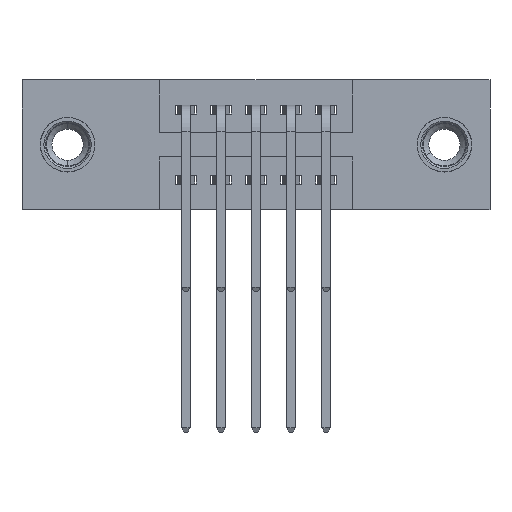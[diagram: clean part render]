
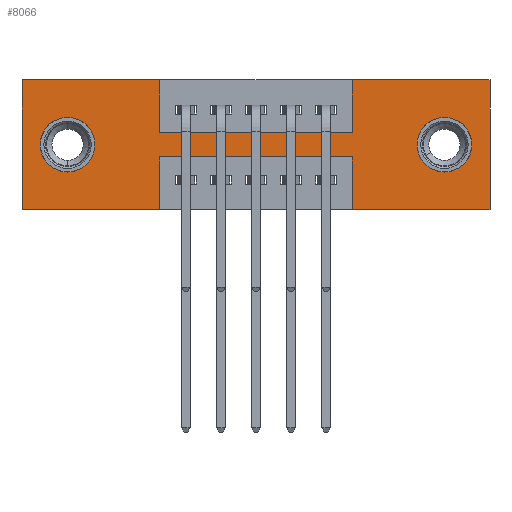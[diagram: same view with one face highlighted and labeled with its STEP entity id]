
A CAD part, front view. The second image highlights one B-rep face of the part: STEP entity #8066.
In plain terms, the highlighted planar face has unit normal (0, -1, 0).
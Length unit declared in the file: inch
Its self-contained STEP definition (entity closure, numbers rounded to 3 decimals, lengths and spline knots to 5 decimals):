
#124 = CARTESIAN_POINT ( 'NONE',  ( 0.13, 0., -0.107 ) ) ;
#285 = EDGE_CURVE ( 'NONE', #5624, #4382, #314, .T. ) ;
#314 = LINE ( 'NONE', #6345, #8420 ) ;
#387 = ORIENTED_EDGE ( 'NONE', *, *, #9266, .F. ) ;
#446 = CARTESIAN_POINT ( 'NONE',  ( 1.335, 0., 0. ) ) ;
#456 = VECTOR ( 'NONE', #890, 39.37008 ) ;
#556 = EDGE_CURVE ( 'NONE', #1943, #1924, #5445, .T. ) ;
#660 = CARTESIAN_POINT ( 'NONE',  ( 0.13, 0., -0.185 ) ) ;
#846 = LINE ( 'NONE', #3126, #1568 ) ;
#890 = DIRECTION ( 'NONE',  ( 0., 0., -1. ) ) ;
#943 = CIRCLE ( 'NONE', #5551, 0.078 ) ;
#991 = AXIS2_PLACEMENT_3D ( 'NONE', #660, #4293, #2564 ) ;
#1037 = CARTESIAN_POINT ( 'NONE',  ( 1.205, 0., -0.107 ) ) ;
#1059 = ORIENTED_EDGE ( 'NONE', *, *, #285, .F. ) ;
#1102 = EDGE_CURVE ( 'NONE', #2141, #6295, #6740, .T. ) ;
#1112 = LINE ( 'NONE', #446, #1966 ) ;
#1154 = DIRECTION ( 'NONE',  ( 0., 0., -1. ) ) ;
#1337 = ORIENTED_EDGE ( 'NONE', *, *, #6542, .F. ) ;
#1438 = CIRCLE ( 'NONE', #5416, 0.078 ) ;
#1516 = VERTEX_POINT ( 'NONE', #3893 ) ;
#1568 = VECTOR ( 'NONE', #9356, 39.37008 ) ;
#1778 = CARTESIAN_POINT ( 'NONE',  ( 0.9425, 0., -0.37 ) ) ;
#1865 = LINE ( 'NONE', #2783, #8841 ) ;
#1924 = VERTEX_POINT ( 'NONE', #8941 ) ;
#1943 = VERTEX_POINT ( 'NONE', #9131 ) ;
#1966 = VECTOR ( 'NONE', #10240, 39.37008 ) ;
#2069 = DIRECTION ( 'NONE',  ( -1., 0., 0. ) ) ;
#2093 = CARTESIAN_POINT ( 'NONE',  ( 0., 0., -0.37 ) ) ;
#2141 = VERTEX_POINT ( 'NONE', #4515 ) ;
#2258 = ORIENTED_EDGE ( 'NONE', *, *, #6096, .F. ) ;
#2370 = EDGE_CURVE ( 'NONE', #5806, #4892, #2661, .T. ) ;
#2421 = EDGE_CURVE ( 'NONE', #6821, #2141, #6537, .T. ) ;
#2564 = DIRECTION ( 'NONE',  ( 0., 0., 1. ) ) ;
#2661 = LINE ( 'NONE', #6543, #5100 ) ;
#2773 = DIRECTION ( 'NONE',  ( -1., 0., 0. ) ) ;
#2783 = CARTESIAN_POINT ( 'NONE',  ( 0.3925, 0., -0.15 ) ) ;
#2960 = VERTEX_POINT ( 'NONE', #124 ) ;
#2991 = VECTOR ( 'NONE', #6778, 39.37008 ) ;
#3007 = DIRECTION ( 'NONE',  ( -1., 0., 0. ) ) ;
#3012 = EDGE_CURVE ( 'NONE', #11773, #7939, #943, .T. ) ;
#3013 = VECTOR ( 'NONE', #3007, 39.37008 ) ;
#3015 = CARTESIAN_POINT ( 'NONE',  ( 1.205, 0., -0.185 ) ) ;
#3053 = CARTESIAN_POINT ( 'NONE',  ( 0.9425, 0., -0.37 ) ) ;
#3126 = CARTESIAN_POINT ( 'NONE',  ( 0., 0., 0. ) ) ;
#3303 = CARTESIAN_POINT ( 'NONE',  ( 0.3925, 0., -0.37 ) ) ;
#3607 = CARTESIAN_POINT ( 'NONE',  ( 0., 0., 0. ) ) ;
#3664 = EDGE_LOOP ( 'NONE', ( #7920, #7869 ) ) ;
#3737 = CARTESIAN_POINT ( 'NONE',  ( 0.13, 0., -0.185 ) ) ;
#3795 = ORIENTED_EDGE ( 'NONE', *, *, #1102, .F. ) ;
#3893 = CARTESIAN_POINT ( 'NONE',  ( 0.9425, 0., -0.15 ) ) ;
#3914 = DIRECTION ( 'NONE',  ( 0., -1., 0. ) ) ;
#3948 = VECTOR ( 'NONE', #6461, 39.37008 ) ;
#4037 = CARTESIAN_POINT ( 'NONE',  ( 0.9425, 0., 0. ) ) ;
#4293 = DIRECTION ( 'NONE',  ( 0., 1., 0. ) ) ;
#4382 = VERTEX_POINT ( 'NONE', #7331 ) ;
#4403 = AXIS2_PLACEMENT_3D ( 'NONE', #3737, #4655, #6509 ) ;
#4515 = CARTESIAN_POINT ( 'NONE',  ( 0.3925, 0., 0. ) ) ;
#4655 = DIRECTION ( 'NONE',  ( 0., 1., 0. ) ) ;
#4892 = VERTEX_POINT ( 'NONE', #5484 ) ;
#5100 = VECTOR ( 'NONE', #2773, 39.37008 ) ;
#5107 = VECTOR ( 'NONE', #8743, 39.37008 ) ;
#5134 = VERTEX_POINT ( 'NONE', #6933 ) ;
#5219 = EDGE_CURVE ( 'NONE', #7484, #2960, #8994, .T. ) ;
#5242 = DIRECTION ( 'NONE',  ( 0., 1., 0. ) ) ;
#5380 = DIRECTION ( 'NONE',  ( 1., 0., 0. ) ) ;
#5416 = AXIS2_PLACEMENT_3D ( 'NONE', #3015, #6614, #1154 ) ;
#5428 = VECTOR ( 'NONE', #2069, 39.37008 ) ;
#5433 = CARTESIAN_POINT ( 'NONE',  ( 0.3925, 0., 0. ) ) ;
#5445 = LINE ( 'NONE', #2093, #3013 ) ;
#5484 = CARTESIAN_POINT ( 'NONE',  ( 0.3925, 0., -0.22 ) ) ;
#5500 = VERTEX_POINT ( 'NONE', #1778 ) ;
#5508 = CARTESIAN_POINT ( 'NONE',  ( 0.3925, 0., -0.15 ) ) ;
#5551 = AXIS2_PLACEMENT_3D ( 'NONE', #10126, #5242, #7912 ) ;
#5624 = VERTEX_POINT ( 'NONE', #4037 ) ;
#5806 = VERTEX_POINT ( 'NONE', #10615 ) ;
#6044 = LINE ( 'NONE', #3053, #2991 ) ;
#6096 = EDGE_CURVE ( 'NONE', #6295, #1516, #1865, .T. ) ;
#6206 = EDGE_CURVE ( 'NONE', #5134, #5500, #7138, .T. ) ;
#6295 = VERTEX_POINT ( 'NONE', #5508 ) ;
#6345 = CARTESIAN_POINT ( 'NONE',  ( 0., 0., 0. ) ) ;
#6406 = ORIENTED_EDGE ( 'NONE', *, *, #9818, .F. ) ;
#6461 = DIRECTION ( 'NONE',  ( 1., 0., 0. ) ) ;
#6485 = ORIENTED_EDGE ( 'NONE', *, *, #5219, .T. ) ;
#6509 = DIRECTION ( 'NONE',  ( 0., 0., 1. ) ) ;
#6537 = LINE ( 'NONE', #3607, #3948 ) ;
#6542 = EDGE_CURVE ( 'NONE', #5500, #5806, #6044, .T. ) ;
#6543 = CARTESIAN_POINT ( 'NONE',  ( 0.3925, 0., -0.22 ) ) ;
#6576 = EDGE_CURVE ( 'NONE', #7939, #11773, #1438, .T. ) ;
#6614 = DIRECTION ( 'NONE',  ( 0., 1., 0. ) ) ;
#6740 = LINE ( 'NONE', #5433, #456 ) ;
#6778 = DIRECTION ( 'NONE',  ( 0., 0., 1. ) ) ;
#6821 = VERTEX_POINT ( 'NONE', #7726 ) ;
#6854 = DIRECTION ( 'NONE',  ( 0., 0., 1. ) ) ;
#6933 = CARTESIAN_POINT ( 'NONE',  ( 1.335, 0., -0.37 ) ) ;
#6958 = ORIENTED_EDGE ( 'NONE', *, *, #7185, .F. ) ;
#7138 = LINE ( 'NONE', #10275, #5428 ) ;
#7185 = EDGE_CURVE ( 'NONE', #1516, #5624, #9655, .T. ) ;
#7257 = FACE_BOUND ( 'NONE', #3664, .T. ) ;
#7331 = CARTESIAN_POINT ( 'NONE',  ( 1.335, 0., 0. ) ) ;
#7484 = VERTEX_POINT ( 'NONE', #10761 ) ;
#7496 = DIRECTION ( 'NONE',  ( 1., 0., 0. ) ) ;
#7726 = CARTESIAN_POINT ( 'NONE',  ( 0., 0., 0. ) ) ;
#7869 = ORIENTED_EDGE ( 'NONE', *, *, #3012, .T. ) ;
#7912 = DIRECTION ( 'NONE',  ( 0., 0., -1. ) ) ;
#7919 = ORIENTED_EDGE ( 'NONE', *, *, #2421, .F. ) ;
#7920 = ORIENTED_EDGE ( 'NONE', *, *, #6576, .T. ) ;
#7939 = VERTEX_POINT ( 'NONE', #1037 ) ;
#7968 = EDGE_LOOP ( 'NONE', ( #8078, #10206, #1337, #10150, #6406, #1059, #6958, #2258, #3795, #7919, #387, #8931 ) ) ;
#8066 = ADVANCED_FACE ( 'NONE', ( #7257, #9521, #9789 ), #10930, .T. ) ;
#8078 = ORIENTED_EDGE ( 'NONE', *, *, #9881, .F. ) ;
#8324 = EDGE_LOOP ( 'NONE', ( #10879, #6485 ) ) ;
#8420 = VECTOR ( 'NONE', #5380, 39.37008 ) ;
#8511 = LINE ( 'NONE', #3303, #5107 ) ;
#8513 = CARTESIAN_POINT ( 'NONE',  ( 0., 0., -0.37 ) ) ;
#8592 = CARTESIAN_POINT ( 'NONE',  ( 1.205, 0., -0.263 ) ) ;
#8743 = DIRECTION ( 'NONE',  ( 0., 0., -1. ) ) ;
#8775 = EDGE_CURVE ( 'NONE', #2960, #7484, #9673, .T. ) ;
#8841 = VECTOR ( 'NONE', #7496, 39.37008 ) ;
#8931 = ORIENTED_EDGE ( 'NONE', *, *, #556, .F. ) ;
#8941 = CARTESIAN_POINT ( 'NONE',  ( 0., 0., -0.37 ) ) ;
#8994 = CIRCLE ( 'NONE', #991, 0.078 ) ;
#9107 = AXIS2_PLACEMENT_3D ( 'NONE', #8513, #3914, #10247 ) ;
#9131 = CARTESIAN_POINT ( 'NONE',  ( 0.3925, 0., -0.37 ) ) ;
#9266 = EDGE_CURVE ( 'NONE', #1924, #6821, #846, .T. ) ;
#9356 = DIRECTION ( 'NONE',  ( 0., 0., 1. ) ) ;
#9373 = VECTOR ( 'NONE', #6854, 39.37008 ) ;
#9521 = FACE_BOUND ( 'NONE', #8324, .T. ) ;
#9655 = LINE ( 'NONE', #10347, #9373 ) ;
#9673 = CIRCLE ( 'NONE', #4403, 0.078 ) ;
#9789 = FACE_OUTER_BOUND ( 'NONE', #7968, .T. ) ;
#9818 = EDGE_CURVE ( 'NONE', #4382, #5134, #1112, .T. ) ;
#9881 = EDGE_CURVE ( 'NONE', #4892, #1943, #8511, .T. ) ;
#10126 = CARTESIAN_POINT ( 'NONE',  ( 1.205, 0., -0.185 ) ) ;
#10150 = ORIENTED_EDGE ( 'NONE', *, *, #6206, .F. ) ;
#10206 = ORIENTED_EDGE ( 'NONE', *, *, #2370, .F. ) ;
#10240 = DIRECTION ( 'NONE',  ( 0., 0., -1. ) ) ;
#10247 = DIRECTION ( 'NONE',  ( 0., 0., -1. ) ) ;
#10275 = CARTESIAN_POINT ( 'NONE',  ( 0., 0., -0.37 ) ) ;
#10347 = CARTESIAN_POINT ( 'NONE',  ( 0.9425, 0., 0. ) ) ;
#10615 = CARTESIAN_POINT ( 'NONE',  ( 0.9425, 0., -0.22 ) ) ;
#10761 = CARTESIAN_POINT ( 'NONE',  ( 0.13, 0., -0.263 ) ) ;
#10879 = ORIENTED_EDGE ( 'NONE', *, *, #8775, .T. ) ;
#10930 = PLANE ( 'NONE',  #9107 ) ;
#11773 = VERTEX_POINT ( 'NONE', #8592 ) ;
